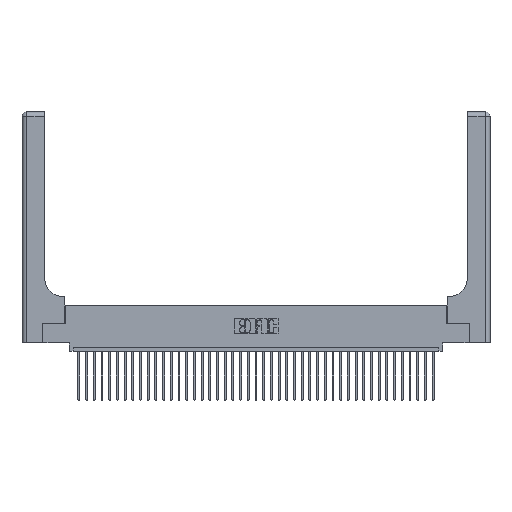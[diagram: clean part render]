
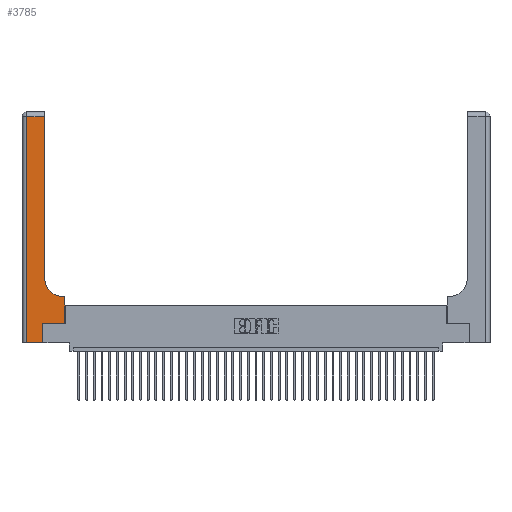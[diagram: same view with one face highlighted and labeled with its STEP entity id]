
A CAD part, top view. The second image highlights one B-rep face of the part: STEP entity #3785.
In plain terms, the highlighted planar face has unit normal (0, 0, 1).
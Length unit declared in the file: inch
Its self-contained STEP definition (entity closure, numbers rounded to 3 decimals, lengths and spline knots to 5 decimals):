
#42 = CIRCLE ( 'NONE', #21933, 0.25 ) ;
#361 = LINE ( 'NONE', #978, #2812 ) ;
#978 = CARTESIAN_POINT ( 'NONE',  ( 0.2915, 0.6, 0.37 ) ) ;
#1537 = LINE ( 'NONE', #5049, #25641 ) ;
#2377 = DIRECTION ( 'NONE',  ( 0., -1., 0. ) ) ;
#2812 = VECTOR ( 'NONE', #19838, 39.37008 ) ;
#2837 = DIRECTION ( 'NONE',  ( 1., 0., 0. ) ) ;
#3169 = ORIENTED_EDGE ( 'NONE', *, *, #3882, .T. ) ;
#3785 = ADVANCED_FACE ( 'NONE', ( #24288 ), #8382, .F. ) ;
#3882 = EDGE_CURVE ( 'NONE', #20936, #7258, #36890, .T. ) ;
#4544 = VERTEX_POINT ( 'NONE', #39885 ) ;
#5049 = CARTESIAN_POINT ( 'NONE',  ( 0.06, 3., 0.37 ) ) ;
#5088 = ORIENTED_EDGE ( 'NONE', *, *, #16667, .T. ) ;
#5399 = VECTOR ( 'NONE', #7483, 39.37008 ) ;
#7258 = VERTEX_POINT ( 'NONE', #31977 ) ;
#7380 = DIRECTION ( 'NONE',  ( 0., 0., -1. ) ) ;
#7483 = DIRECTION ( 'NONE',  ( -1., 0., 0. ) ) ;
#7783 = VERTEX_POINT ( 'NONE', #17257 ) ;
#7925 = CARTESIAN_POINT ( 'NONE',  ( 0.5585, 0.25, 0.37 ) ) ;
#8189 = AXIS2_PLACEMENT_3D ( 'NONE', #14601, #30009, #33118 ) ;
#8382 = PLANE ( 'NONE',  #8189 ) ;
#9082 = VERTEX_POINT ( 'NONE', #12193 ) ;
#10476 = LINE ( 'NONE', #30512, #28893 ) ;
#10715 = VERTEX_POINT ( 'NONE', #33701 ) ;
#12193 = CARTESIAN_POINT ( 'NONE',  ( 0.5585, 0.25, 0.37 ) ) ;
#14135 = DIRECTION ( 'NONE',  ( 1., 0., 0. ) ) ;
#14473 = ORIENTED_EDGE ( 'NONE', *, *, #17263, .T. ) ;
#14601 = CARTESIAN_POINT ( 'NONE',  ( 0., 3., 0.37 ) ) ;
#14725 = VERTEX_POINT ( 'NONE', #34494 ) ;
#14852 = VERTEX_POINT ( 'NONE', #23563 ) ;
#14964 = DIRECTION ( 'NONE',  ( 1., 0., 0. ) ) ;
#15570 = VECTOR ( 'NONE', #30823, 39.37008 ) ;
#16522 = LINE ( 'NONE', #28097, #15570 ) ;
#16638 = ORIENTED_EDGE ( 'NONE', *, *, #36085, .T. ) ;
#16667 = EDGE_CURVE ( 'NONE', #7258, #20510, #37862, .T. ) ;
#17238 = ORIENTED_EDGE ( 'NONE', *, *, #34253, .T. ) ;
#17257 = CARTESIAN_POINT ( 'NONE',  ( 0.5415, 0.6, 0.37 ) ) ;
#17263 = EDGE_CURVE ( 'NONE', #10715, #4544, #16522, .T. ) ;
#19296 = EDGE_CURVE ( 'NONE', #7783, #10715, #42, .T. ) ;
#19838 = DIRECTION ( 'NONE',  ( -1., 0., 0. ) ) ;
#19982 = CARTESIAN_POINT ( 'NONE',  ( 0.269, 0., 0.37 ) ) ;
#20074 = CARTESIAN_POINT ( 'NONE',  ( 0.06, 0., 0.37 ) ) ;
#20510 = VERTEX_POINT ( 'NONE', #32578 ) ;
#20580 = EDGE_LOOP ( 'NONE', ( #14473, #38726, #16638, #3169, #5088, #39563, #17238, #36922, #38835 ) ) ;
#20936 = VERTEX_POINT ( 'NONE', #20074 ) ;
#21385 = VECTOR ( 'NONE', #35428, 39.37008 ) ;
#21933 = AXIS2_PLACEMENT_3D ( 'NONE', #38746, #7380, #14135 ) ;
#23003 = DIRECTION ( 'NONE',  ( 0., 1., 0. ) ) ;
#23563 = CARTESIAN_POINT ( 'NONE',  ( 0.5585, 0.6, 0.37 ) ) ;
#24288 = FACE_OUTER_BOUND ( 'NONE', #20580, .T. ) ;
#25641 = VECTOR ( 'NONE', #2377, 39.37008 ) ;
#25902 = CARTESIAN_POINT ( 'NONE',  ( 0., 0., 0.37 ) ) ;
#26212 = VECTOR ( 'NONE', #14964, 39.37008 ) ;
#28097 = CARTESIAN_POINT ( 'NONE',  ( 0.2915, 3., 0.37 ) ) ;
#28893 = VECTOR ( 'NONE', #2837, 39.37008 ) ;
#29035 = EDGE_CURVE ( 'NONE', #20510, #9082, #10476, .T. ) ;
#29473 = EDGE_CURVE ( 'NONE', #14852, #7783, #361, .T. ) ;
#30009 = DIRECTION ( 'NONE',  ( 0., 0., -1. ) ) ;
#30512 = CARTESIAN_POINT ( 'NONE',  ( 0.269, 0.25, 0.37 ) ) ;
#30823 = DIRECTION ( 'NONE',  ( 0., 1., 0. ) ) ;
#31977 = CARTESIAN_POINT ( 'NONE',  ( 0.269, 0., 0.37 ) ) ;
#32578 = CARTESIAN_POINT ( 'NONE',  ( 0.269, 0.25, 0.37 ) ) ;
#33088 = VECTOR ( 'NONE', #23003, 39.37008 ) ;
#33118 = DIRECTION ( 'NONE',  ( -1., 0., 0. ) ) ;
#33701 = CARTESIAN_POINT ( 'NONE',  ( 0.2915, 0.85, 0.37 ) ) ;
#34253 = EDGE_CURVE ( 'NONE', #9082, #14852, #34998, .T. ) ;
#34416 = LINE ( 'NONE', #35329, #5399 ) ;
#34494 = CARTESIAN_POINT ( 'NONE',  ( 0.06, 2.94, 0.37 ) ) ;
#34998 = LINE ( 'NONE', #7925, #33088 ) ;
#35329 = CARTESIAN_POINT ( 'NONE',  ( 0., 2.94, 0.37 ) ) ;
#35428 = DIRECTION ( 'NONE',  ( 0., 1., 0. ) ) ;
#35973 = EDGE_CURVE ( 'NONE', #4544, #14725, #34416, .T. ) ;
#36085 = EDGE_CURVE ( 'NONE', #14725, #20936, #1537, .T. ) ;
#36890 = LINE ( 'NONE', #25902, #26212 ) ;
#36922 = ORIENTED_EDGE ( 'NONE', *, *, #29473, .T. ) ;
#37862 = LINE ( 'NONE', #19982, #21385 ) ;
#38726 = ORIENTED_EDGE ( 'NONE', *, *, #35973, .T. ) ;
#38746 = CARTESIAN_POINT ( 'NONE',  ( 0.5415, 0.85, 0.37 ) ) ;
#38835 = ORIENTED_EDGE ( 'NONE', *, *, #19296, .T. ) ;
#39563 = ORIENTED_EDGE ( 'NONE', *, *, #29035, .T. ) ;
#39885 = CARTESIAN_POINT ( 'NONE',  ( 0.2915, 2.94, 0.37 ) ) ;
